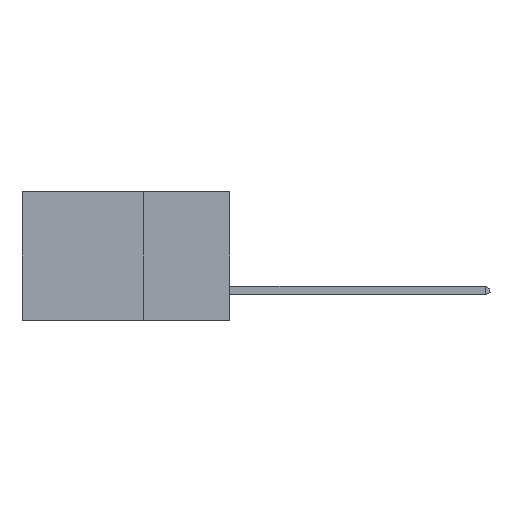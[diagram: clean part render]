
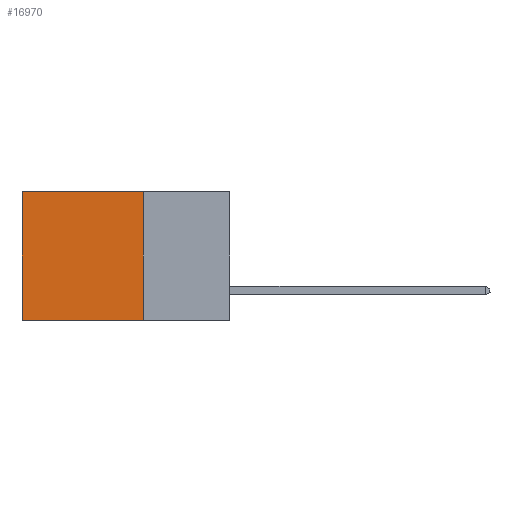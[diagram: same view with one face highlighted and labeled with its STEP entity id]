
A CAD part, left-side view. The second image highlights one B-rep face of the part: STEP entity #16970.
In plain terms, the highlighted planar face has unit normal (-1, 0, 0).
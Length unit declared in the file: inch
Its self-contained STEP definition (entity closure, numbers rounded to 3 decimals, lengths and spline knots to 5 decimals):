
#1637 = CARTESIAN_POINT ( 'NONE',  ( 0.298, 0.25, 0. ) ) ;
#1919 = CARTESIAN_POINT ( 'NONE',  ( 0.298, 0.25, 0. ) ) ;
#1928 = LINE ( 'NONE', #24349, #16601 ) ;
#2755 = VERTEX_POINT ( 'NONE', #15599 ) ;
#2839 = LINE ( 'NONE', #22870, #14732 ) ;
#3628 = EDGE_CURVE ( 'NONE', #2755, #3960, #2839, .T. ) ;
#3960 = VERTEX_POINT ( 'NONE', #17694 ) ;
#4938 = LINE ( 'NONE', #15327, #14084 ) ;
#5550 = CARTESIAN_POINT ( 'NONE',  ( 0.298, 0.25, 0. ) ) ;
#6583 = VECTOR ( 'NONE', #26963, 39.37008 ) ;
#6915 = EDGE_CURVE ( 'NONE', #13071, #12696, #9756, .T. ) ;
#8064 = DIRECTION ( 'NONE',  ( 0., 0., -1. ) ) ;
#9756 = LINE ( 'NONE', #1637, #6583 ) ;
#11876 = FACE_OUTER_BOUND ( 'NONE', #14219, .T. ) ;
#12333 = DIRECTION ( 'NONE',  ( 0., 1., 0. ) ) ;
#12696 = VERTEX_POINT ( 'NONE', #20665 ) ;
#13071 = VERTEX_POINT ( 'NONE', #1919 ) ;
#14084 = VECTOR ( 'NONE', #14373, 39.37008 ) ;
#14219 = EDGE_LOOP ( 'NONE', ( #27216, #15884, #30230, #19480 ) ) ;
#14373 = DIRECTION ( 'NONE',  ( 0., 1., 0. ) ) ;
#14732 = VECTOR ( 'NONE', #32829, 39.37008 ) ;
#15327 = CARTESIAN_POINT ( 'NONE',  ( 0.298, 0.25, 0. ) ) ;
#15599 = CARTESIAN_POINT ( 'NONE',  ( 0.298, 0.6, 0. ) ) ;
#15884 = ORIENTED_EDGE ( 'NONE', *, *, #32391, .F. ) ;
#16601 = VECTOR ( 'NONE', #12333, 39.37008 ) ;
#16970 = ADVANCED_FACE ( 'NONE', ( #11876 ), #20504, .F. ) ;
#17694 = CARTESIAN_POINT ( 'NONE',  ( 0.298, 0.6, -0.37 ) ) ;
#18064 = DIRECTION ( 'NONE',  ( 1., 0., 0. ) ) ;
#19480 = ORIENTED_EDGE ( 'NONE', *, *, #27231, .T. ) ;
#20504 = PLANE ( 'NONE',  #22246 ) ;
#20665 = CARTESIAN_POINT ( 'NONE',  ( 0.298, 0.25, -0.37 ) ) ;
#22246 = AXIS2_PLACEMENT_3D ( 'NONE', #5550, #18064, #8064 ) ;
#22870 = CARTESIAN_POINT ( 'NONE',  ( 0.298, 0.6, 0. ) ) ;
#24349 = CARTESIAN_POINT ( 'NONE',  ( 0.298, 0.25, -0.37 ) ) ;
#26963 = DIRECTION ( 'NONE',  ( 0., 0., -1. ) ) ;
#27216 = ORIENTED_EDGE ( 'NONE', *, *, #3628, .T. ) ;
#27231 = EDGE_CURVE ( 'NONE', #13071, #2755, #4938, .T. ) ;
#30230 = ORIENTED_EDGE ( 'NONE', *, *, #6915, .F. ) ;
#32391 = EDGE_CURVE ( 'NONE', #12696, #3960, #1928, .T. ) ;
#32829 = DIRECTION ( 'NONE',  ( 0., 0., -1. ) ) ;
